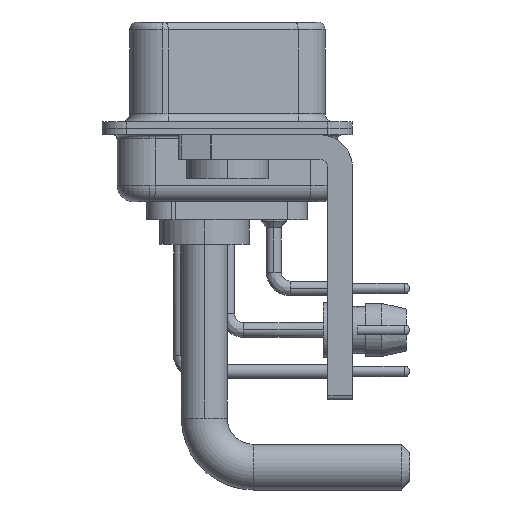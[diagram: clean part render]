
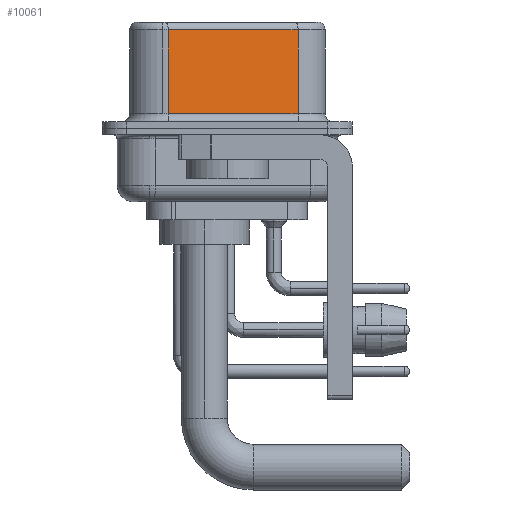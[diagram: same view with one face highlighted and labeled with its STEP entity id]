
A CAD part, left-side view. The second image highlights one B-rep face of the part: STEP entity #10061.
In plain terms, the highlighted planar face has unit normal (-0.985, -0.174, 0).
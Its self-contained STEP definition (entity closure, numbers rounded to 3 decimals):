
#239 = VECTOR ( 'NONE', #7244, 1000. ) ;
#692 = CARTESIAN_POINT ( 'NONE',  ( 5.132, -4.322, 0.9 ) ) ;
#2538 = CARTESIAN_POINT ( 'NONE',  ( 3.73, 3.628, 6.02 ) ) ;
#4403 = VERTEX_POINT ( 'NONE', #6309 ) ;
#4750 = VECTOR ( 'NONE', #16650, 1000. ) ;
#6309 = CARTESIAN_POINT ( 'NONE',  ( 5.132, -4.322, 6.02 ) ) ;
#7244 = DIRECTION ( 'NONE',  ( -0.174, 0.985, 0. ) ) ;
#8149 = DIRECTION ( 'NONE',  ( 0., 0., -1. ) ) ;
#9472 = VERTEX_POINT ( 'NONE', #17295 ) ;
#9604 = EDGE_CURVE ( 'NONE', #4403, #13936, #15415, .T. ) ;
#10061 = ADVANCED_FACE ( 'NONE', ( #21129 ), #29312, .F. ) ;
#10098 = EDGE_CURVE ( 'NONE', #9472, #24215, #18712, .T. ) ;
#11774 = ORIENTED_EDGE ( 'NONE', *, *, #26863, .F. ) ;
#13533 = LINE ( 'NONE', #25062, #27856 ) ;
#13894 = LINE ( 'NONE', #18738, #19730 ) ;
#13936 = VERTEX_POINT ( 'NONE', #2538 ) ;
#15203 = ORIENTED_EDGE ( 'NONE', *, *, #34962, .T. ) ;
#15415 = LINE ( 'NONE', #23783, #239 ) ;
#15552 = CARTESIAN_POINT ( 'NONE',  ( 5.132, -4.322, 6.52 ) ) ;
#15737 = DIRECTION ( 'NONE',  ( -0.174, 0.985, 0. ) ) ;
#16650 = DIRECTION ( 'NONE',  ( 0.174, -0.985, 0. ) ) ;
#17295 = CARTESIAN_POINT ( 'NONE',  ( 3.73, 3.628, 0.9 ) ) ;
#18530 = DIRECTION ( 'NONE',  ( 0.985, 0.174, 0. ) ) ;
#18712 = LINE ( 'NONE', #30058, #4750 ) ;
#18738 = CARTESIAN_POINT ( 'NONE',  ( 5.132, -4.322, 6.52 ) ) ;
#19090 = ORIENTED_EDGE ( 'NONE', *, *, #10098, .T. ) ;
#19730 = VECTOR ( 'NONE', #30824, 1000. ) ;
#20080 = EDGE_LOOP ( 'NONE', ( #11774, #36037, #15203, #19090 ) ) ;
#21129 = FACE_OUTER_BOUND ( 'NONE', #20080, .T. ) ;
#23783 = CARTESIAN_POINT ( 'NONE',  ( 5.132, -4.322, 6.02 ) ) ;
#24215 = VERTEX_POINT ( 'NONE', #692 ) ;
#25062 = CARTESIAN_POINT ( 'NONE',  ( 3.73, 3.628, 6.52 ) ) ;
#26863 = EDGE_CURVE ( 'NONE', #4403, #24215, #13894, .T. ) ;
#27342 = AXIS2_PLACEMENT_3D ( 'NONE', #15552, #18530, #15737 ) ;
#27856 = VECTOR ( 'NONE', #8149, 1000. ) ;
#29312 = PLANE ( 'NONE',  #27342 ) ;
#30058 = CARTESIAN_POINT ( 'NONE',  ( 5.132, -4.322, 0.9 ) ) ;
#30824 = DIRECTION ( 'NONE',  ( 0., 0., -1. ) ) ;
#34962 = EDGE_CURVE ( 'NONE', #13936, #9472, #13533, .T. ) ;
#36037 = ORIENTED_EDGE ( 'NONE', *, *, #9604, .T. ) ;
